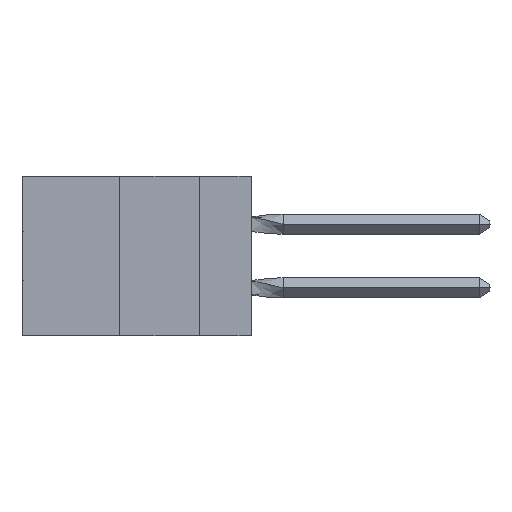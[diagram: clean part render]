
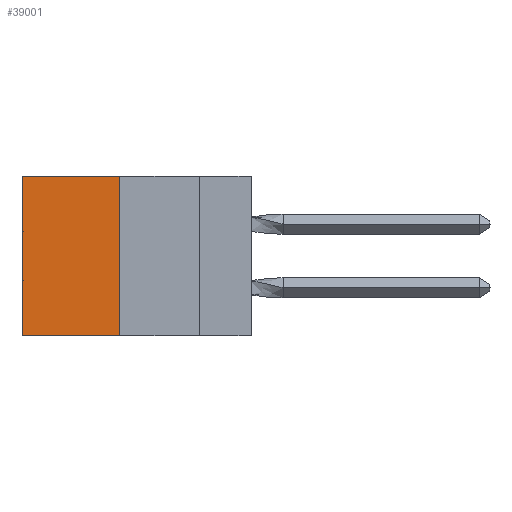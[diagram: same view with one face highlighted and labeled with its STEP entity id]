
A CAD part, left-side view. The second image highlights one B-rep face of the part: STEP entity #39001.
In plain terms, the highlighted planar face has unit normal (-1, 0, 0).
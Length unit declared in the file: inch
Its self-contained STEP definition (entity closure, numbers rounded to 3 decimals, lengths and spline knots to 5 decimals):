
#496 = VECTOR ( 'NONE', #19373, 39.37008 ) ;
#1548 = EDGE_CURVE ( 'NONE', #28463, #12176, #38816, .T. ) ;
#3005 = CARTESIAN_POINT ( 'NONE',  ( 0.305, 0.413, 0. ) ) ;
#3861 = CARTESIAN_POINT ( 'NONE',  ( 0.305, 0.413, -0.5 ) ) ;
#5399 = FACE_OUTER_BOUND ( 'NONE', #31253, .T. ) ;
#6706 = CARTESIAN_POINT ( 'NONE',  ( 0.305, 0.413, -0.5 ) ) ;
#7405 = DIRECTION ( 'NONE',  ( 0., 0., -1. ) ) ;
#7442 = DIRECTION ( 'NONE',  ( 0., 0., -1. ) ) ;
#7547 = VERTEX_POINT ( 'NONE', #13013 ) ;
#8703 = EDGE_CURVE ( 'NONE', #28463, #27583, #19284, .T. ) ;
#8714 = ORIENTED_EDGE ( 'NONE', *, *, #10358, .T. ) ;
#10028 = CARTESIAN_POINT ( 'NONE',  ( 0.305, 0.72, 0. ) ) ;
#10358 = EDGE_CURVE ( 'NONE', #12176, #7547, #12706, .T. ) ;
#12176 = VERTEX_POINT ( 'NONE', #10028 ) ;
#12247 = VECTOR ( 'NONE', #34419, 39.37008 ) ;
#12706 = LINE ( 'NONE', #29562, #496 ) ;
#13013 = CARTESIAN_POINT ( 'NONE',  ( 0.305, 0.72, -0.5 ) ) ;
#19284 = LINE ( 'NONE', #6706, #41595 ) ;
#19373 = DIRECTION ( 'NONE',  ( 0., 0., -1. ) ) ;
#20700 = LINE ( 'NONE', #29621, #30774 ) ;
#22126 = AXIS2_PLACEMENT_3D ( 'NONE', #3861, #30969, #7442 ) ;
#24151 = PLANE ( 'NONE',  #22126 ) ;
#26854 = ORIENTED_EDGE ( 'NONE', *, *, #1548, .T. ) ;
#27583 = VERTEX_POINT ( 'NONE', #30364 ) ;
#27639 = CARTESIAN_POINT ( 'NONE',  ( 0.305, 0.413, 0. ) ) ;
#28463 = VERTEX_POINT ( 'NONE', #3005 ) ;
#29562 = CARTESIAN_POINT ( 'NONE',  ( 0.305, 0.72, -0.5 ) ) ;
#29621 = CARTESIAN_POINT ( 'NONE',  ( 0.305, 0.413, -0.5 ) ) ;
#30364 = CARTESIAN_POINT ( 'NONE',  ( 0.305, 0.413, -0.5 ) ) ;
#30774 = VECTOR ( 'NONE', #40392, 39.37008 ) ;
#30969 = DIRECTION ( 'NONE',  ( 1., 0., 0. ) ) ;
#31253 = EDGE_LOOP ( 'NONE', ( #8714, #32241, #43495, #26854 ) ) ;
#32241 = ORIENTED_EDGE ( 'NONE', *, *, #35714, .F. ) ;
#34419 = DIRECTION ( 'NONE',  ( 0., 1., 0. ) ) ;
#35714 = EDGE_CURVE ( 'NONE', #27583, #7547, #20700, .T. ) ;
#38816 = LINE ( 'NONE', #27639, #12247 ) ;
#39001 = ADVANCED_FACE ( 'NONE', ( #5399 ), #24151, .F. ) ;
#40392 = DIRECTION ( 'NONE',  ( 0., 1., 0. ) ) ;
#41595 = VECTOR ( 'NONE', #7405, 39.37008 ) ;
#43495 = ORIENTED_EDGE ( 'NONE', *, *, #8703, .F. ) ;
